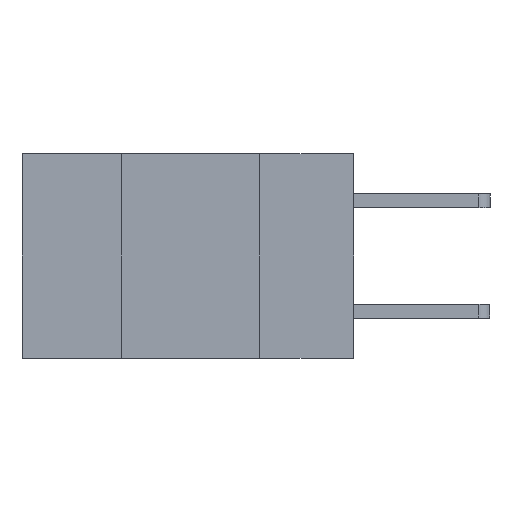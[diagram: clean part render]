
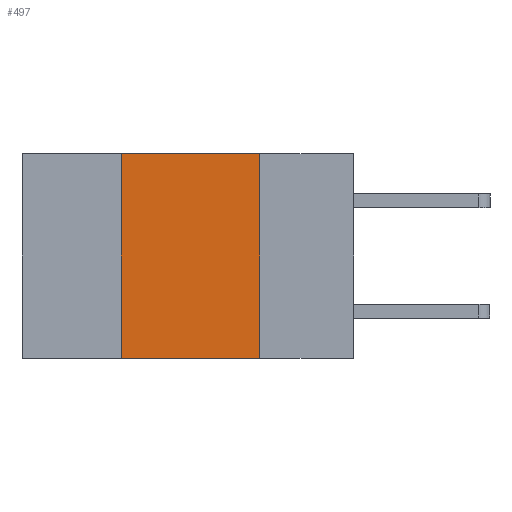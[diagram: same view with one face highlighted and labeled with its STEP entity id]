
A CAD part, left-side view. The second image highlights one B-rep face of the part: STEP entity #497.
In plain terms, the highlighted planar face has unit normal (-1, 0, 0).
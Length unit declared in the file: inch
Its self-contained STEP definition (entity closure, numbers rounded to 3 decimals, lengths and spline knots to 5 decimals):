
#142 = CARTESIAN_POINT ( 'NONE',  ( 0., 0.17, 0. ) ) ;
#191 = LINE ( 'NONE', #142, #1467 ) ;
#387 = ORIENTED_EDGE ( 'NONE', *, *, #6647, .T. ) ;
#497 = ADVANCED_FACE ( 'NONE', ( #2591 ), #5931, .F. ) ;
#633 = DIRECTION ( 'NONE',  ( 1., 0., 0. ) ) ;
#777 = CARTESIAN_POINT ( 'NONE',  ( 0., 0.42, 0. ) ) ;
#978 = VERTEX_POINT ( 'NONE', #777 ) ;
#1364 = VECTOR ( 'NONE', #3680, 39.37008 ) ;
#1430 = LINE ( 'NONE', #5442, #2401 ) ;
#1467 = VECTOR ( 'NONE', #10211, 39.37008 ) ;
#1573 = CARTESIAN_POINT ( 'NONE',  ( 0., 0.42, -0.37 ) ) ;
#1984 = EDGE_CURVE ( 'NONE', #8679, #9421, #191, .T. ) ;
#2003 = CARTESIAN_POINT ( 'NONE',  ( 0., 0.6, -0.37 ) ) ;
#2177 = DIRECTION ( 'NONE',  ( 0., -1., 0. ) ) ;
#2341 = EDGE_LOOP ( 'NONE', ( #10784, #10200, #6246, #387 ) ) ;
#2401 = VECTOR ( 'NONE', #8801, 39.37008 ) ;
#2591 = FACE_OUTER_BOUND ( 'NONE', #2341, .T. ) ;
#2793 = CARTESIAN_POINT ( 'NONE',  ( 0., 0.17, -0.37 ) ) ;
#3680 = DIRECTION ( 'NONE',  ( 0., -1., 0. ) ) ;
#4072 = CARTESIAN_POINT ( 'NONE',  ( 0., 0.6, 0. ) ) ;
#4747 = LINE ( 'NONE', #6341, #8084 ) ;
#4905 = CARTESIAN_POINT ( 'NONE',  ( 0., 0.17, 0. ) ) ;
#5109 = EDGE_CURVE ( 'NONE', #5775, #978, #1430, .T. ) ;
#5442 = CARTESIAN_POINT ( 'NONE',  ( 0., 0.42, 0. ) ) ;
#5775 = VERTEX_POINT ( 'NONE', #1573 ) ;
#5931 = PLANE ( 'NONE',  #9171 ) ;
#6246 = ORIENTED_EDGE ( 'NONE', *, *, #5109, .F. ) ;
#6341 = CARTESIAN_POINT ( 'NONE',  ( 0., 0.6, 0. ) ) ;
#6647 = EDGE_CURVE ( 'NONE', #5775, #9421, #10382, .T. ) ;
#7996 = EDGE_CURVE ( 'NONE', #978, #8679, #4747, .T. ) ;
#8084 = VECTOR ( 'NONE', #2177, 39.37008 ) ;
#8679 = VERTEX_POINT ( 'NONE', #4905 ) ;
#8801 = DIRECTION ( 'NONE',  ( 0., 0., 1. ) ) ;
#9171 = AXIS2_PLACEMENT_3D ( 'NONE', #4072, #633, #9302 ) ;
#9302 = DIRECTION ( 'NONE',  ( 0., 0., -1. ) ) ;
#9421 = VERTEX_POINT ( 'NONE', #2793 ) ;
#10200 = ORIENTED_EDGE ( 'NONE', *, *, #7996, .F. ) ;
#10211 = DIRECTION ( 'NONE',  ( 0., 0., -1. ) ) ;
#10382 = LINE ( 'NONE', #2003, #1364 ) ;
#10784 = ORIENTED_EDGE ( 'NONE', *, *, #1984, .F. ) ;
